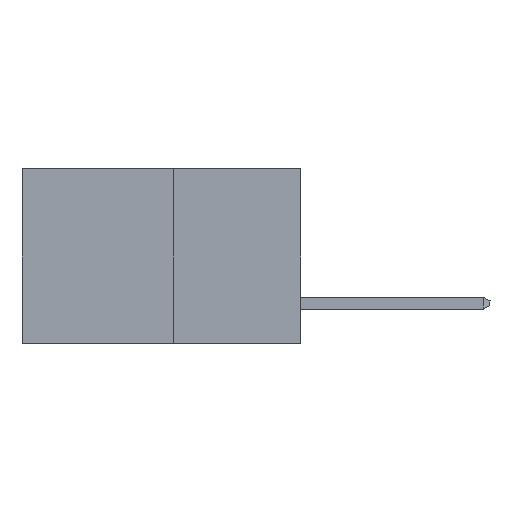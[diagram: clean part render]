
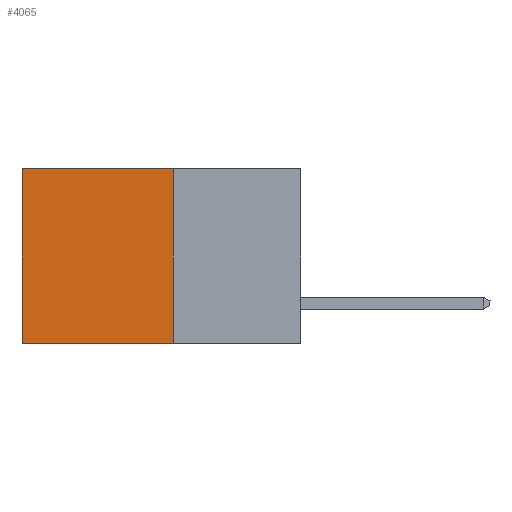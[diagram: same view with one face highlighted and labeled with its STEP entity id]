
A CAD part, left-side view. The second image highlights one B-rep face of the part: STEP entity #4065.
In plain terms, the highlighted planar face has unit normal (-1, 0, 0).
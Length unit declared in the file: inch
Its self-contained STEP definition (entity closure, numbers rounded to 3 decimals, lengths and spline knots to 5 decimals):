
#417 = LINE ( 'NONE', #14813, #15184 ) ;
#719 = VERTEX_POINT ( 'NONE', #17337 ) ;
#796 = CARTESIAN_POINT ( 'NONE',  ( 0.277, 0.27, -0.37 ) ) ;
#939 = EDGE_CURVE ( 'NONE', #15874, #719, #1125, .T. ) ;
#1125 = LINE ( 'NONE', #14909, #12106 ) ;
#2041 = EDGE_CURVE ( 'NONE', #719, #9143, #17843, .T. ) ;
#2054 = DIRECTION ( 'NONE',  ( 0., 0., -1. ) ) ;
#2153 = EDGE_CURVE ( 'NONE', #5904, #9143, #417, .T. ) ;
#2224 = VECTOR ( 'NONE', #11818, 39.37008 ) ;
#2537 = VECTOR ( 'NONE', #17470, 39.37008 ) ;
#4065 = ADVANCED_FACE ( 'NONE', ( #14235 ), #18235, .F. ) ;
#4754 = ORIENTED_EDGE ( 'NONE', *, *, #2041, .F. ) ;
#5904 = VERTEX_POINT ( 'NONE', #5933 ) ;
#5933 = CARTESIAN_POINT ( 'NONE',  ( 0.277, 0.59, 0. ) ) ;
#6189 = CARTESIAN_POINT ( 'NONE',  ( 0.277, 0.27, 0. ) ) ;
#8528 = AXIS2_PLACEMENT_3D ( 'NONE', #796, #18232, #18175 ) ;
#9143 = VERTEX_POINT ( 'NONE', #9342 ) ;
#9342 = CARTESIAN_POINT ( 'NONE',  ( 0.277, 0.59, -0.37 ) ) ;
#10193 = LINE ( 'NONE', #6189, #2537 ) ;
#11818 = DIRECTION ( 'NONE',  ( 0., 1., 0. ) ) ;
#11992 = EDGE_LOOP ( 'NONE', ( #16336, #4754, #12949, #15746 ) ) ;
#12106 = VECTOR ( 'NONE', #2054, 39.37008 ) ;
#12949 = ORIENTED_EDGE ( 'NONE', *, *, #939, .F. ) ;
#13306 = DIRECTION ( 'NONE',  ( 0., 0., -1. ) ) ;
#14235 = FACE_OUTER_BOUND ( 'NONE', #11992, .T. ) ;
#14813 = CARTESIAN_POINT ( 'NONE',  ( 0.277, 0.59, -0.37 ) ) ;
#14909 = CARTESIAN_POINT ( 'NONE',  ( 0.277, 0.27, -0.37 ) ) ;
#15171 = CARTESIAN_POINT ( 'NONE',  ( 0.277, 0.27, 0. ) ) ;
#15184 = VECTOR ( 'NONE', #13306, 39.37008 ) ;
#15608 = EDGE_CURVE ( 'NONE', #15874, #5904, #10193, .T. ) ;
#15746 = ORIENTED_EDGE ( 'NONE', *, *, #15608, .T. ) ;
#15874 = VERTEX_POINT ( 'NONE', #15171 ) ;
#16263 = CARTESIAN_POINT ( 'NONE',  ( 0.277, 0.27, -0.37 ) ) ;
#16336 = ORIENTED_EDGE ( 'NONE', *, *, #2153, .T. ) ;
#17337 = CARTESIAN_POINT ( 'NONE',  ( 0.277, 0.27, -0.37 ) ) ;
#17470 = DIRECTION ( 'NONE',  ( 0., 1., 0. ) ) ;
#17843 = LINE ( 'NONE', #16263, #2224 ) ;
#18175 = DIRECTION ( 'NONE',  ( 0., 0., -1. ) ) ;
#18232 = DIRECTION ( 'NONE',  ( 1., 0., 0. ) ) ;
#18235 = PLANE ( 'NONE',  #8528 ) ;
